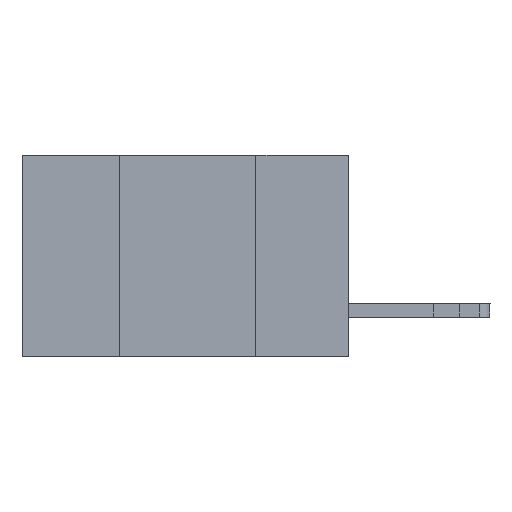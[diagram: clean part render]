
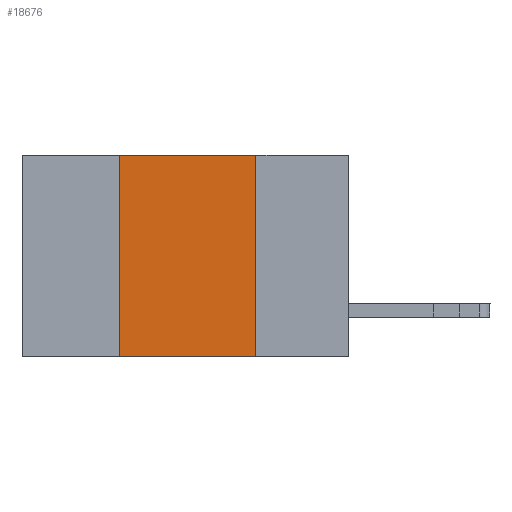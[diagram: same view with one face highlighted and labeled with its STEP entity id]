
A CAD part, left-side view. The second image highlights one B-rep face of the part: STEP entity #18676.
In plain terms, the highlighted planar face has unit normal (-1, 0, 0).
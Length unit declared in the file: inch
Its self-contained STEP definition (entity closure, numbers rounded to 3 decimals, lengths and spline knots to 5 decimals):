
#280 = VERTEX_POINT ( 'NONE', #14799 ) ;
#288 = CARTESIAN_POINT ( 'NONE',  ( 0., 0.42, -0.37 ) ) ;
#753 = LINE ( 'NONE', #17462, #12776 ) ;
#1082 = AXIS2_PLACEMENT_3D ( 'NONE', #12813, #8140, #12921 ) ;
#1816 = VERTEX_POINT ( 'NONE', #11406 ) ;
#2640 = CARTESIAN_POINT ( 'NONE',  ( 0., 0.42, 0. ) ) ;
#3133 = DIRECTION ( 'NONE',  ( 0., 0., -1. ) ) ;
#3149 = CARTESIAN_POINT ( 'NONE',  ( 0., 0.6, -0.37 ) ) ;
#3595 = VERTEX_POINT ( 'NONE', #8823 ) ;
#4504 = VECTOR ( 'NONE', #11699, 39.37008 ) ;
#5307 = CARTESIAN_POINT ( 'NONE',  ( 0., 0.17, 0. ) ) ;
#6099 = ORIENTED_EDGE ( 'NONE', *, *, #17634, .T. ) ;
#6316 = ORIENTED_EDGE ( 'NONE', *, *, #14611, .F. ) ;
#6931 = FACE_OUTER_BOUND ( 'NONE', #8573, .T. ) ;
#7641 = VECTOR ( 'NONE', #3133, 39.37008 ) ;
#7716 = DIRECTION ( 'NONE',  ( 0., 0., 1. ) ) ;
#8140 = DIRECTION ( 'NONE',  ( 1., 0., 0. ) ) ;
#8573 = EDGE_LOOP ( 'NONE', ( #20925, #11136, #6316, #6099 ) ) ;
#8823 = CARTESIAN_POINT ( 'NONE',  ( 0., 0.17, -0.37 ) ) ;
#9691 = EDGE_CURVE ( 'NONE', #280, #3595, #11910, .T. ) ;
#11136 = ORIENTED_EDGE ( 'NONE', *, *, #16739, .F. ) ;
#11406 = CARTESIAN_POINT ( 'NONE',  ( 0., 0.42, 0. ) ) ;
#11699 = DIRECTION ( 'NONE',  ( 0., -1., 0. ) ) ;
#11910 = LINE ( 'NONE', #5307, #7641 ) ;
#12776 = VECTOR ( 'NONE', #14206, 39.37008 ) ;
#12813 = CARTESIAN_POINT ( 'NONE',  ( 0., 0.6, 0. ) ) ;
#12921 = DIRECTION ( 'NONE',  ( 0., 0., -1. ) ) ;
#13011 = LINE ( 'NONE', #3149, #4504 ) ;
#13023 = PLANE ( 'NONE',  #1082 ) ;
#14206 = DIRECTION ( 'NONE',  ( 0., -1., 0. ) ) ;
#14611 = EDGE_CURVE ( 'NONE', #18145, #1816, #17499, .T. ) ;
#14799 = CARTESIAN_POINT ( 'NONE',  ( 0., 0.17, 0. ) ) ;
#15536 = VECTOR ( 'NONE', #7716, 39.37008 ) ;
#16739 = EDGE_CURVE ( 'NONE', #1816, #280, #753, .T. ) ;
#17462 = CARTESIAN_POINT ( 'NONE',  ( 0., 0.6, 0. ) ) ;
#17499 = LINE ( 'NONE', #2640, #15536 ) ;
#17634 = EDGE_CURVE ( 'NONE', #18145, #3595, #13011, .T. ) ;
#18145 = VERTEX_POINT ( 'NONE', #288 ) ;
#18676 = ADVANCED_FACE ( 'NONE', ( #6931 ), #13023, .F. ) ;
#20925 = ORIENTED_EDGE ( 'NONE', *, *, #9691, .F. ) ;
